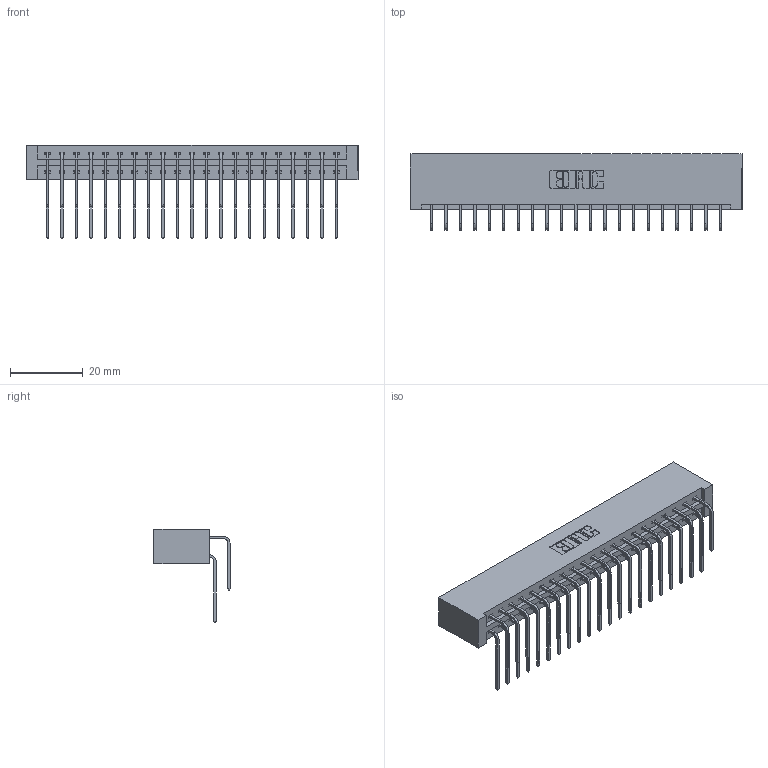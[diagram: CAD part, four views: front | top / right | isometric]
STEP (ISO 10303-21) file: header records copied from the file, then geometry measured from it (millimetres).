
FILE_DESCRIPTION (( 'STEP AP203' ), '1' );
FILE_NAME ('337-042-559-201.STEP', '2018-08-09T01:51:46', ( '' ), ( '' ), 'SwSTEP 2.0', 'SolidWorks 2016', '' );
FILE_SCHEMA (( 'CONFIG_CONTROL_DESIGN' ));
Length unit declared in the file: inch
Products named in the file (4): 337-042-559-201; 337 Part_No Mounting Lugs; 345-292-001_558 559 Tail - 1; 345-292-001_559 Tail - 2
Assembly tree (43 placements, depth 2):
  337-042-559-201
    337 Part_No Mounting Lugs
    345-292-001_558 559 Tail - 1  x21
    345-292-001_559 Tail - 2  x21
Bounding box: 91.08 x 20.9 x 25.53 mm (x, y, z)
Volume: 10322.7 mm3; surface area: 12738.5 mm2
Topology: 43 solids, 43 shells, 2458 faces, 7301 edges, 4810 vertices
Faces by surface type: plane 1746, cylinder 712
Entity records: 20505 total; most frequent: CARTESIAN_POINT 3517, ORIENTED_EDGE 3402, DIRECTION 3005, EDGE_CURVE 1701, VECTOR 1541, LINE 1541, VERTEX_POINT 1130, AXIS2_PLACEMENT_3D 732
